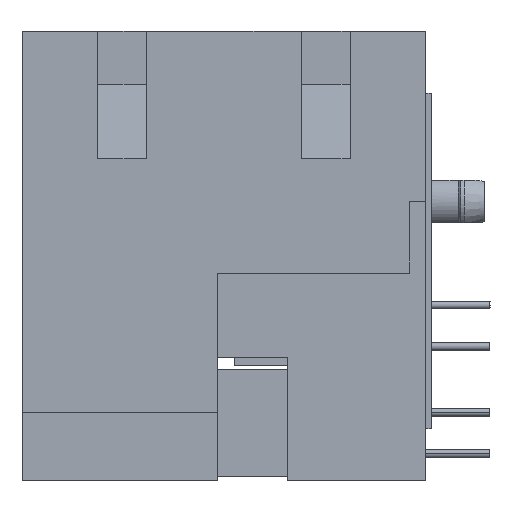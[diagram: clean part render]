
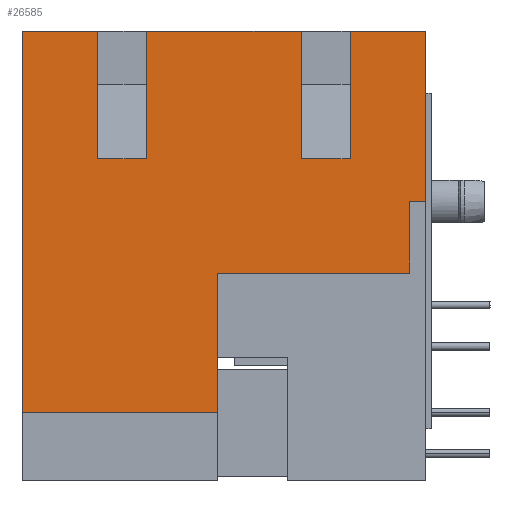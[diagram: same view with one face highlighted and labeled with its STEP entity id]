
A CAD part, left-side view. The second image highlights one B-rep face of the part: STEP entity #26585.
In plain terms, the highlighted planar face has unit normal (-1, 0, 0).
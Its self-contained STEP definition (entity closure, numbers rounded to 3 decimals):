
#932 = CARTESIAN_POINT ( 'NONE',  ( -29.34, 10.839, 13.8 ) ) ;
#1088 = CARTESIAN_POINT ( 'NONE',  ( -29.34, 12.384, -9.6 ) ) ;
#1144 = DIRECTION ( 'NONE',  ( 1., 0., 0. ) ) ;
#1589 = EDGE_CURVE ( 'NONE', #38758, #25488, #14071, .T. ) ;
#1662 = ORIENTED_EDGE ( 'NONE', *, *, #29363, .F. ) ;
#1780 = VERTEX_POINT ( 'NONE', #50008 ) ;
#2564 = B_SPLINE_CURVE_WITH_KNOTS ( 'NONE', 3,
 ( #48249, #26507, #27447, #54016 ),
 .UNSPECIFIED., .F., .F.,
 ( 4, 4 ),
 ( 0., 1. ),
 .UNSPECIFIED. ) ;
#3095 = DIRECTION ( 'NONE',  ( 0., 0., 1. ) ) ;
#3597 = VERTEX_POINT ( 'NONE', #7492 ) ;
#4404 = EDGE_CURVE ( 'NONE', #1780, #30104, #49833, .T. ) ;
#5397 = CARTESIAN_POINT ( 'NONE',  ( -29.34, -4.75, 5.972 ) ) ;
#6426 = CARTESIAN_POINT ( 'NONE',  ( -29.34, -12.384, 13.8 ) ) ;
#6634 = LINE ( 'NONE', #28410, #40162 ) ;
#7093 = DIRECTION ( 'NONE',  ( 0., -1., 0. ) ) ;
#7492 = CARTESIAN_POINT ( 'NONE',  ( -29.34, 0.4, -1.05 ) ) ;
#7495 = LINE ( 'NONE', #55411, #48577 ) ;
#7836 = VECTOR ( 'NONE', #56385, 1000. ) ;
#8480 = CARTESIAN_POINT ( 'NONE',  ( -29.34, 4.75, 2.1 ) ) ;
#9583 = ORIENTED_EDGE ( 'NONE', *, *, #30528, .F. ) ;
#10357 = CARTESIAN_POINT ( 'NONE',  ( -29.34, 7.75, 5.972 ) ) ;
#11049 = VECTOR ( 'NONE', #37253, 1000. ) ;
#11367 = CARTESIAN_POINT ( 'NONE',  ( -29.34, -7.75, 5.972 ) ) ;
#11398 = EDGE_CURVE ( 'NONE', #37788, #1780, #56308, .T. ) ;
#12391 = ORIENTED_EDGE ( 'NONE', *, *, #49141, .F. ) ;
#12409 = LINE ( 'NONE', #23946, #11049 ) ;
#13870 = CARTESIAN_POINT ( 'NONE',  ( -29.34, -12.879, 14.268 ) ) ;
#14071 = LINE ( 'NONE', #21407, #7836 ) ;
#14264 = VECTOR ( 'NONE', #42901, 1000. ) ;
#14680 = VERTEX_POINT ( 'NONE', #21232 ) ;
#14712 = VERTEX_POINT ( 'NONE', #26396 ) ;
#16415 = CARTESIAN_POINT ( 'NONE',  ( -29.34, -10.839, 13.8 ) ) ;
#16949 = LINE ( 'NONE', #24413, #37436 ) ;
#17522 = DIRECTION ( 'NONE',  ( 0., 0., 1. ) ) ;
#17555 = VECTOR ( 'NONE', #31095, 1000. ) ;
#19249 = AXIS2_PLACEMENT_3D ( 'NONE', #13870, #1144, #27441 ) ;
#20829 = EDGE_CURVE ( 'NONE', #35035, #48412, #12409, .T. ) ;
#21232 = CARTESIAN_POINT ( 'NONE',  ( -29.34, -11.4, 3.35 ) ) ;
#21277 = EDGE_CURVE ( 'NONE', #14680, #44624, #53478, .T. ) ;
#21407 = CARTESIAN_POINT ( 'NONE',  ( -29.34, 0., -9.6 ) ) ;
#21438 = ORIENTED_EDGE ( 'NONE', *, *, #20829, .F. ) ;
#21736 = CARTESIAN_POINT ( 'NONE',  ( -29.34, 12.383, 2.1 ) ) ;
#21969 = VERTEX_POINT ( 'NONE', #55817 ) ;
#22092 = ORIENTED_EDGE ( 'NONE', *, *, #48127, .F. ) ;
#23084 = EDGE_CURVE ( 'NONE', #44624, #3597, #29381, .T. ) ;
#23591 = CARTESIAN_POINT ( 'NONE',  ( -29.34, 9.294, 13.8 ) ) ;
#23719 = LINE ( 'NONE', #48453, #17555 ) ;
#23879 = CARTESIAN_POINT ( 'NONE',  ( -29.34, -11.4, 2.1 ) ) ;
#23936 = VECTOR ( 'NONE', #46643, 1000. ) ;
#23946 = CARTESIAN_POINT ( 'NONE',  ( -29.34, -4.75, 2.1 ) ) ;
#24062 = ORIENTED_EDGE ( 'NONE', *, *, #52904, .F. ) ;
#24413 = CARTESIAN_POINT ( 'NONE',  ( -29.34, 7.75, 2.1 ) ) ;
#24621 = ORIENTED_EDGE ( 'NONE', *, *, #11398, .T. ) ;
#24686 = CARTESIAN_POINT ( 'NONE',  ( -29.34, -4.75, 13.8 ) ) ;
#25488 = VERTEX_POINT ( 'NONE', #1088 ) ;
#26226 = CARTESIAN_POINT ( 'NONE',  ( -29.34, 0.4, -9.6 ) ) ;
#26272 = CARTESIAN_POINT ( 'NONE',  ( -29.34, 7.75, 13.8 ) ) ;
#26396 = CARTESIAN_POINT ( 'NONE',  ( -29.34, 12.383, 13.8 ) ) ;
#26507 = CARTESIAN_POINT ( 'NONE',  ( -29.34, -1.583, 13.8 ) ) ;
#26585 = ADVANCED_FACE ( 'NONE', ( #47385 ), #44395, .F. ) ;
#27228 = CARTESIAN_POINT ( 'NONE',  ( -29.34, 7.75, 13.8 ) ) ;
#27441 = DIRECTION ( 'NONE',  ( 0., 0., -1. ) ) ;
#27447 = CARTESIAN_POINT ( 'NONE',  ( -29.34, 1.583, 13.8 ) ) ;
#27501 = EDGE_CURVE ( 'NONE', #25488, #14712, #54254, .T. ) ;
#27881 = DIRECTION ( 'NONE',  ( 0., 0., -1. ) ) ;
#27961 = DIRECTION ( 'NONE',  ( 0., 1., 0. ) ) ;
#28410 = CARTESIAN_POINT ( 'NONE',  ( -29.34, 0., 5.972 ) ) ;
#28928 = EDGE_CURVE ( 'NONE', #21969, #33655, #36767, .T. ) ;
#29363 = EDGE_CURVE ( 'NONE', #33448, #21969, #6634, .T. ) ;
#29381 = LINE ( 'NONE', #42418, #23936 ) ;
#29389 = EDGE_CURVE ( 'NONE', #48927, #33448, #16949, .T. ) ;
#29570 = ORIENTED_EDGE ( 'NONE', *, *, #28928, .F. ) ;
#29776 = CARTESIAN_POINT ( 'NONE',  ( -29.34, -7.75, 13.8 ) ) ;
#30104 = VERTEX_POINT ( 'NONE', #52109 ) ;
#30528 = EDGE_CURVE ( 'NONE', #48412, #38155, #46201, .T. ) ;
#31062 = B_SPLINE_CURVE_WITH_KNOTS ( 'NONE', 3,
 ( #27228, #23591, #932, #36149 ),
 .UNSPECIFIED., .F., .F.,
 ( 4, 4 ),
 ( 0., 1. ),
 .UNSPECIFIED. ) ;
#31095 = DIRECTION ( 'NONE',  ( 0., 0., -1. ) ) ;
#32817 = EDGE_LOOP ( 'NONE', ( #35726, #33096, #12391, #24621, #50020, #22092, #9583, #21438, #43513, #29570, #1662, #34347, #34562, #43162, #34452, #24062 ) ) ;
#32969 = DIRECTION ( 'NONE',  ( 0., 0., -1. ) ) ;
#33096 = ORIENTED_EDGE ( 'NONE', *, *, #21277, .F. ) ;
#33448 = VERTEX_POINT ( 'NONE', #10357 ) ;
#33655 = VERTEX_POINT ( 'NONE', #34777 ) ;
#34244 = CARTESIAN_POINT ( 'NONE',  ( -29.34, 0., 5.972 ) ) ;
#34347 = ORIENTED_EDGE ( 'NONE', *, *, #29389, .F. ) ;
#34452 = ORIENTED_EDGE ( 'NONE', *, *, #1589, .F. ) ;
#34562 = ORIENTED_EDGE ( 'NONE', *, *, #38346, .T. ) ;
#34777 = CARTESIAN_POINT ( 'NONE',  ( -29.34, 4.75, 13.8 ) ) ;
#34903 = CARTESIAN_POINT ( 'NONE',  ( -29.34, -11.4, -1.05 ) ) ;
#35035 = VERTEX_POINT ( 'NONE', #24686 ) ;
#35726 = ORIENTED_EDGE ( 'NONE', *, *, #23084, .F. ) ;
#36149 = CARTESIAN_POINT ( 'NONE',  ( -29.34, 12.383, 13.8 ) ) ;
#36767 = LINE ( 'NONE', #8480, #14264 ) ;
#37253 = DIRECTION ( 'NONE',  ( 0., 0., -1. ) ) ;
#37436 = VECTOR ( 'NONE', #32969, 1000. ) ;
#37788 = VERTEX_POINT ( 'NONE', #39276 ) ;
#38155 = VERTEX_POINT ( 'NONE', #11367 ) ;
#38346 = EDGE_CURVE ( 'NONE', #48927, #14712, #31062, .T. ) ;
#38639 = DIRECTION ( 'NONE',  ( 0., -1., 0. ) ) ;
#38758 = VERTEX_POINT ( 'NONE', #26226 ) ;
#39276 = CARTESIAN_POINT ( 'NONE',  ( -29.34, -12.384, 3.35 ) ) ;
#40162 = VECTOR ( 'NONE', #7093, 1000. ) ;
#42418 = CARTESIAN_POINT ( 'NONE',  ( -29.34, 0., -1.05 ) ) ;
#42539 = VECTOR ( 'NONE', #17522, 1000. ) ;
#42901 = DIRECTION ( 'NONE',  ( 0., 0., 1. ) ) ;
#42952 = VECTOR ( 'NONE', #27961, 1000. ) ;
#43162 = ORIENTED_EDGE ( 'NONE', *, *, #27501, .F. ) ;
#43256 = EDGE_CURVE ( 'NONE', #35035, #33655, #2564, .T. ) ;
#43513 = ORIENTED_EDGE ( 'NONE', *, *, #43256, .T. ) ;
#43583 = CARTESIAN_POINT ( 'NONE',  ( -29.34, -12.384, 0. ) ) ;
#44395 = PLANE ( 'NONE',  #19249 ) ;
#44472 = DIRECTION ( 'NONE',  ( 0., 0., 1. ) ) ;
#44624 = VERTEX_POINT ( 'NONE', #34903 ) ;
#45844 = CARTESIAN_POINT ( 'NONE',  ( -29.34, 0., 3.35 ) ) ;
#46201 = LINE ( 'NONE', #34244, #56518 ) ;
#46643 = DIRECTION ( 'NONE',  ( 0., 1., 0. ) ) ;
#47385 = FACE_OUTER_BOUND ( 'NONE', #32817, .T. ) ;
#48127 = EDGE_CURVE ( 'NONE', #38155, #30104, #7495, .T. ) ;
#48249 = CARTESIAN_POINT ( 'NONE',  ( -29.34, -4.75, 13.8 ) ) ;
#48412 = VERTEX_POINT ( 'NONE', #5397 ) ;
#48453 = CARTESIAN_POINT ( 'NONE',  ( -29.34, 0.4, 2.1 ) ) ;
#48577 = VECTOR ( 'NONE', #3095, 1000. ) ;
#48927 = VERTEX_POINT ( 'NONE', #26272 ) ;
#49141 = EDGE_CURVE ( 'NONE', #37788, #14680, #55302, .T. ) ;
#49322 = VECTOR ( 'NONE', #27881, 1000. ) ;
#49833 = B_SPLINE_CURVE_WITH_KNOTS ( 'NONE', 3,
 ( #6426, #16415, #51557, #29776 ),
 .UNSPECIFIED., .F., .F.,
 ( 4, 4 ),
 ( 0., 1. ),
 .UNSPECIFIED. ) ;
#50008 = CARTESIAN_POINT ( 'NONE',  ( -29.34, -12.384, 13.8 ) ) ;
#50020 = ORIENTED_EDGE ( 'NONE', *, *, #4404, .T. ) ;
#50802 = VECTOR ( 'NONE', #44472, 1000. ) ;
#51557 = CARTESIAN_POINT ( 'NONE',  ( -29.34, -9.295, 13.8 ) ) ;
#52109 = CARTESIAN_POINT ( 'NONE',  ( -29.34, -7.75, 13.8 ) ) ;
#52904 = EDGE_CURVE ( 'NONE', #3597, #38758, #23719, .T. ) ;
#53478 = LINE ( 'NONE', #23879, #49322 ) ;
#54016 = CARTESIAN_POINT ( 'NONE',  ( -29.34, 4.75, 13.8 ) ) ;
#54254 = LINE ( 'NONE', #21736, #42539 ) ;
#55302 = LINE ( 'NONE', #45844, #42952 ) ;
#55411 = CARTESIAN_POINT ( 'NONE',  ( -29.34, -7.75, 2.1 ) ) ;
#55817 = CARTESIAN_POINT ( 'NONE',  ( -29.34, 4.75, 5.972 ) ) ;
#56308 = LINE ( 'NONE', #43583, #50802 ) ;
#56385 = DIRECTION ( 'NONE',  ( 0., 1., 0. ) ) ;
#56518 = VECTOR ( 'NONE', #38639, 1000. ) ;
